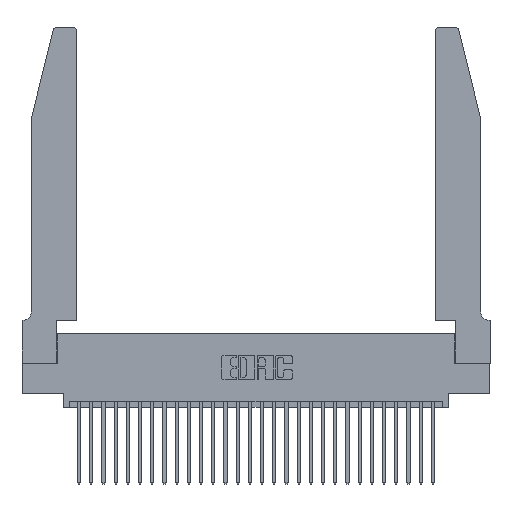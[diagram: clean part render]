
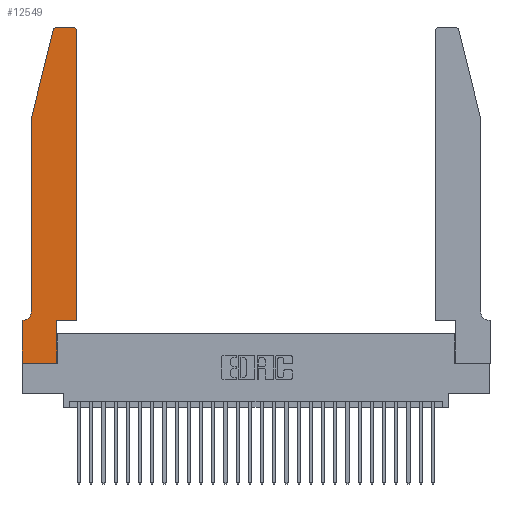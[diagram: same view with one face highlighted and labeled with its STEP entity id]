
A CAD part, top view. The second image highlights one B-rep face of the part: STEP entity #12549.
In plain terms, the highlighted planar face has unit normal (0, 0, 1).
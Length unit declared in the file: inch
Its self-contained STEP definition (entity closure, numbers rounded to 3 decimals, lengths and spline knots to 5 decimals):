
#6 = DIRECTION ( 'NONE',  ( 1., 0., 0. ) ) ;
#238 = LINE ( 'NONE', #7557, #10441 ) ;
#298 = DIRECTION ( 'NONE',  ( 0., 0., 1. ) ) ;
#757 = LINE ( 'NONE', #26107, #24784 ) ;
#1434 = LINE ( 'NONE', #16551, #19609 ) ;
#1439 = CARTESIAN_POINT ( 'NONE',  ( 0.4505, 0.35, 0.37 ) ) ;
#1442 = ORIENTED_EDGE ( 'NONE', *, *, #18246, .T. ) ;
#1494 = ORIENTED_EDGE ( 'NONE', *, *, #25530, .T. ) ;
#1736 = DIRECTION ( 'NONE',  ( 1., 0., 0. ) ) ;
#1823 = DIRECTION ( 'NONE',  ( 0., 0., 1. ) ) ;
#2108 = VERTEX_POINT ( 'NONE', #29302 ) ;
#2174 = FACE_OUTER_BOUND ( 'NONE', #4492, .T. ) ;
#2414 = DIRECTION ( 'NONE',  ( 0., -1., 0. ) ) ;
#2550 = VERTEX_POINT ( 'NONE', #21020 ) ;
#3663 = LINE ( 'NONE', #21577, #27622 ) ;
#3951 = CIRCLE ( 'NONE', #14542, 0.07 ) ;
#4083 = CIRCLE ( 'NONE', #6435, 0.03 ) ;
#4492 = EDGE_LOOP ( 'NONE', ( #1442, #1494, #21332, #12723, #5617, #4793, #12465, #23308, #15081, #16220, #27760, #12199 ) ) ;
#4540 = EDGE_CURVE ( 'NONE', #11441, #2550, #1434, .T. ) ;
#4793 = ORIENTED_EDGE ( 'NONE', *, *, #22378, .T. ) ;
#5617 = ORIENTED_EDGE ( 'NONE', *, *, #28845, .T. ) ;
#5887 = VERTEX_POINT ( 'NONE', #17394 ) ;
#6336 = EDGE_CURVE ( 'NONE', #8496, #2108, #15861, .T. ) ;
#6435 = AXIS2_PLACEMENT_3D ( 'NONE', #19025, #298, #6 ) ;
#6596 = CARTESIAN_POINT ( 'NONE',  ( 0.2865, 0.35, 0.37 ) ) ;
#6633 = DIRECTION ( 'NONE',  ( 1., 0., 0. ) ) ;
#7265 = DIRECTION ( 'NONE',  ( -1., 0., 0. ) ) ;
#7557 = CARTESIAN_POINT ( 'NONE',  ( 0.0755, 2., 0.37 ) ) ;
#7792 = LINE ( 'NONE', #22949, #14378 ) ;
#8097 = EDGE_CURVE ( 'NONE', #12646, #8496, #23105, .T. ) ;
#8496 = VERTEX_POINT ( 'NONE', #21471 ) ;
#8709 = AXIS2_PLACEMENT_3D ( 'NONE', #22511, #1823, #1736 ) ;
#8743 = PLANE ( 'NONE',  #8709 ) ;
#8977 = DIRECTION ( 'NONE',  ( -1., 0., 0. ) ) ;
#9512 = VERTEX_POINT ( 'NONE', #17019 ) ;
#9709 = DIRECTION ( 'NONE',  ( 0., 0., -1. ) ) ;
#10149 = CARTESIAN_POINT ( 'NONE',  ( 0.0755, 0.42, 0.37 ) ) ;
#10441 = VECTOR ( 'NONE', #23756, 39.37008 ) ;
#11441 = VERTEX_POINT ( 'NONE', #26589 ) ;
#11660 = CIRCLE ( 'NONE', #20390, 0.03 ) ;
#12036 = EDGE_CURVE ( 'NONE', #2108, #5887, #11660, .T. ) ;
#12063 = LINE ( 'NONE', #25824, #23014 ) ;
#12145 = VECTOR ( 'NONE', #17714, 39.37008 ) ;
#12199 = ORIENTED_EDGE ( 'NONE', *, *, #12036, .T. ) ;
#12465 = ORIENTED_EDGE ( 'NONE', *, *, #4540, .T. ) ;
#12505 = DIRECTION ( 'NONE',  ( 0., -1., 0. ) ) ;
#12549 = ADVANCED_FACE ( 'NONE', ( #2174 ), #8743, .T. ) ;
#12646 = VERTEX_POINT ( 'NONE', #6596 ) ;
#12688 = CARTESIAN_POINT ( 'NONE',  ( 0.2865, 0., 0.37 ) ) ;
#12723 = ORIENTED_EDGE ( 'NONE', *, *, #13292, .T. ) ;
#13292 = EDGE_CURVE ( 'NONE', #17468, #21411, #3663, .T. ) ;
#13546 = CARTESIAN_POINT ( 'NONE',  ( 0.0055, 0.35, 0.37 ) ) ;
#14378 = VECTOR ( 'NONE', #8977, 39.37008 ) ;
#14469 = DIRECTION ( 'NONE',  ( 0., 1., 0. ) ) ;
#14529 = DIRECTION ( 'NONE',  ( -1., 0., 0. ) ) ;
#14542 = AXIS2_PLACEMENT_3D ( 'NONE', #21313, #9709, #7265 ) ;
#14897 = EDGE_CURVE ( 'NONE', #9512, #17468, #238, .T. ) ;
#15081 = ORIENTED_EDGE ( 'NONE', *, *, #25774, .T. ) ;
#15139 = VECTOR ( 'NONE', #29766, 39.37008 ) ;
#15410 = CARTESIAN_POINT ( 'NONE',  ( 0.4205, 2.72, 0.37 ) ) ;
#15751 = CARTESIAN_POINT ( 'NONE',  ( 0.0755, 2., 0.37 ) ) ;
#15861 = LINE ( 'NONE', #18339, #15139 ) ;
#15884 = LINE ( 'NONE', #24012, #28219 ) ;
#16220 = ORIENTED_EDGE ( 'NONE', *, *, #8097, .T. ) ;
#16551 = CARTESIAN_POINT ( 'NONE',  ( 0., 0., 0.37 ) ) ;
#17019 = CARTESIAN_POINT ( 'NONE',  ( 0.25487, 2.72718, 0.37 ) ) ;
#17394 = CARTESIAN_POINT ( 'NONE',  ( 0.4205, 2.75, 0.37 ) ) ;
#17468 = VERTEX_POINT ( 'NONE', #15751 ) ;
#17470 = CARTESIAN_POINT ( 'NONE',  ( 0.284, 2.75, 0.37 ) ) ;
#17714 = DIRECTION ( 'NONE',  ( 1., 0., 0. ) ) ;
#18246 = EDGE_CURVE ( 'NONE', #5887, #26376, #12063, .T. ) ;
#18339 = CARTESIAN_POINT ( 'NONE',  ( 0.4505, 0.35, 0.37 ) ) ;
#19025 = CARTESIAN_POINT ( 'NONE',  ( 0.284, 2.72, 0.37 ) ) ;
#19609 = VECTOR ( 'NONE', #2414, 39.37008 ) ;
#20390 = AXIS2_PLACEMENT_3D ( 'NONE', #15410, #29471, #6633 ) ;
#20761 = VERTEX_POINT ( 'NONE', #12688 ) ;
#21020 = CARTESIAN_POINT ( 'NONE',  ( 0., 0., 0.37 ) ) ;
#21313 = CARTESIAN_POINT ( 'NONE',  ( 0.0055, 0.42, 0.37 ) ) ;
#21332 = ORIENTED_EDGE ( 'NONE', *, *, #14897, .T. ) ;
#21411 = VERTEX_POINT ( 'NONE', #10149 ) ;
#21471 = CARTESIAN_POINT ( 'NONE',  ( 0.4505, 0.35, 0.37 ) ) ;
#21577 = CARTESIAN_POINT ( 'NONE',  ( 0.0755, 2., 0.37 ) ) ;
#22378 = EDGE_CURVE ( 'NONE', #24006, #11441, #7792, .T. ) ;
#22511 = CARTESIAN_POINT ( 'NONE',  ( 0., 0.35, 0.37 ) ) ;
#22949 = CARTESIAN_POINT ( 'NONE',  ( 0.0755, 0.35, 0.37 ) ) ;
#23014 = VECTOR ( 'NONE', #14529, 39.37008 ) ;
#23105 = LINE ( 'NONE', #1439, #12145 ) ;
#23308 = ORIENTED_EDGE ( 'NONE', *, *, #29799, .T. ) ;
#23756 = DIRECTION ( 'NONE',  ( -0.239, -0.971, 0. ) ) ;
#24006 = VERTEX_POINT ( 'NONE', #13546 ) ;
#24012 = CARTESIAN_POINT ( 'NONE',  ( 0., 0., 0.37 ) ) ;
#24784 = VECTOR ( 'NONE', #14469, 39.37008 ) ;
#24890 = DIRECTION ( 'NONE',  ( 1., 0., 0. ) ) ;
#25530 = EDGE_CURVE ( 'NONE', #26376, #9512, #4083, .T. ) ;
#25774 = EDGE_CURVE ( 'NONE', #20761, #12646, #757, .T. ) ;
#25824 = CARTESIAN_POINT ( 'NONE',  ( 0.2605, 2.75, 0.37 ) ) ;
#26107 = CARTESIAN_POINT ( 'NONE',  ( 0.2865, 0.35, 0.37 ) ) ;
#26376 = VERTEX_POINT ( 'NONE', #17470 ) ;
#26589 = CARTESIAN_POINT ( 'NONE',  ( 0., 0.35, 0.37 ) ) ;
#27622 = VECTOR ( 'NONE', #12505, 39.37008 ) ;
#27760 = ORIENTED_EDGE ( 'NONE', *, *, #6336, .T. ) ;
#28219 = VECTOR ( 'NONE', #24890, 39.37008 ) ;
#28845 = EDGE_CURVE ( 'NONE', #21411, #24006, #3951, .T. ) ;
#29302 = CARTESIAN_POINT ( 'NONE',  ( 0.4505, 2.72, 0.37 ) ) ;
#29471 = DIRECTION ( 'NONE',  ( 0., 0., 1. ) ) ;
#29766 = DIRECTION ( 'NONE',  ( 0., 1., 0. ) ) ;
#29799 = EDGE_CURVE ( 'NONE', #2550, #20761, #15884, .T. ) ;
